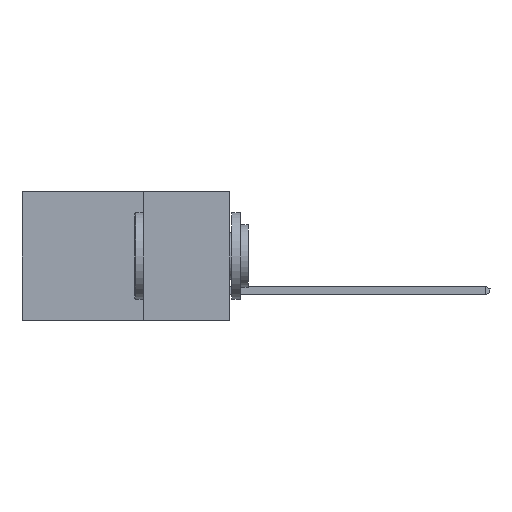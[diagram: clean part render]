
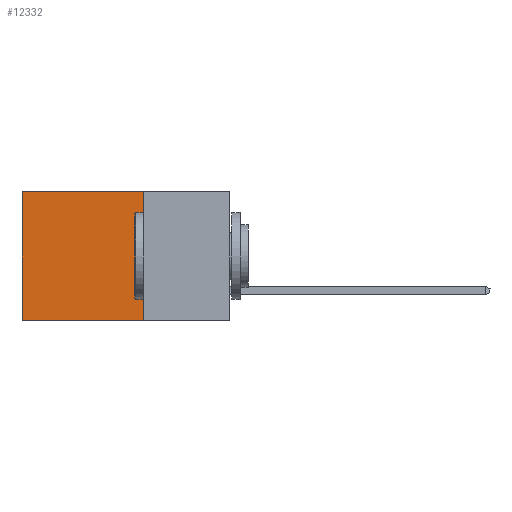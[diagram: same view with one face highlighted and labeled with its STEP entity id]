
A CAD part, left-side view. The second image highlights one B-rep face of the part: STEP entity #12332.
In plain terms, the highlighted planar face has unit normal (-1, 0, 0).
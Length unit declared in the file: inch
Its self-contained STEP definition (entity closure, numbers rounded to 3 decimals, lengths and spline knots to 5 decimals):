
#1079 = CARTESIAN_POINT ( 'NONE',  ( 0.2615, 0.25, -0.37 ) ) ;
#1252 = CARTESIAN_POINT ( 'NONE',  ( 0.2615, 0.25, -0.37 ) ) ;
#1641 = LINE ( 'NONE', #26148, #18589 ) ;
#2982 = PLANE ( 'NONE',  #16964 ) ;
#4997 = VERTEX_POINT ( 'NONE', #24973 ) ;
#5472 = EDGE_CURVE ( 'NONE', #20245, #6253, #1641, .T. ) ;
#5738 = DIRECTION ( 'NONE',  ( 0., 0., -1. ) ) ;
#5756 = ORIENTED_EDGE ( 'NONE', *, *, #8278, .T. ) ;
#6253 = VERTEX_POINT ( 'NONE', #12849 ) ;
#7073 = DIRECTION ( 'NONE',  ( 0., 0., -1. ) ) ;
#7515 = DIRECTION ( 'NONE',  ( 0., 1., 0. ) ) ;
#8278 = EDGE_CURVE ( 'NONE', #4997, #11311, #14027, .T. ) ;
#9537 = VECTOR ( 'NONE', #7515, 39.37008 ) ;
#9671 = DIRECTION ( 'NONE',  ( 0., 0., -1. ) ) ;
#10715 = ORIENTED_EDGE ( 'NONE', *, *, #13516, .T. ) ;
#10894 = CARTESIAN_POINT ( 'NONE',  ( 0.2615, 0.25, 0. ) ) ;
#11213 = VECTOR ( 'NONE', #9671, 39.37008 ) ;
#11311 = VERTEX_POINT ( 'NONE', #25356 ) ;
#11585 = VECTOR ( 'NONE', #17299, 39.37008 ) ;
#11894 = EDGE_CURVE ( 'NONE', #6253, #11311, #26143, .T. ) ;
#12332 = ADVANCED_FACE ( 'NONE', ( #25709 ), #2982, .F. ) ;
#12849 = CARTESIAN_POINT ( 'NONE',  ( 0.2615, 0.25, -0.37 ) ) ;
#13257 = EDGE_LOOP ( 'NONE', ( #5756, #15977, #21659, #10715 ) ) ;
#13516 = EDGE_CURVE ( 'NONE', #20245, #4997, #23386, .T. ) ;
#14027 = LINE ( 'NONE', #24476, #11213 ) ;
#15826 = CARTESIAN_POINT ( 'NONE',  ( 0.2615, 0.25, 0. ) ) ;
#15977 = ORIENTED_EDGE ( 'NONE', *, *, #11894, .F. ) ;
#16964 = AXIS2_PLACEMENT_3D ( 'NONE', #1079, #17849, #7073 ) ;
#17299 = DIRECTION ( 'NONE',  ( 0., 1., 0. ) ) ;
#17849 = DIRECTION ( 'NONE',  ( 1., 0., 0. ) ) ;
#18589 = VECTOR ( 'NONE', #5738, 39.37008 ) ;
#20245 = VERTEX_POINT ( 'NONE', #15826 ) ;
#21659 = ORIENTED_EDGE ( 'NONE', *, *, #5472, .F. ) ;
#23386 = LINE ( 'NONE', #10894, #11585 ) ;
#24476 = CARTESIAN_POINT ( 'NONE',  ( 0.2615, 0.6, -0.37 ) ) ;
#24973 = CARTESIAN_POINT ( 'NONE',  ( 0.2615, 0.6, 0. ) ) ;
#25356 = CARTESIAN_POINT ( 'NONE',  ( 0.2615, 0.6, -0.37 ) ) ;
#25709 = FACE_OUTER_BOUND ( 'NONE', #13257, .T. ) ;
#26143 = LINE ( 'NONE', #1252, #9537 ) ;
#26148 = CARTESIAN_POINT ( 'NONE',  ( 0.2615, 0.25, -0.37 ) ) ;
